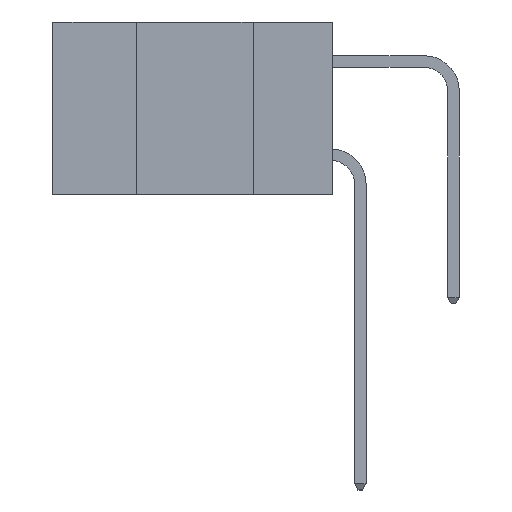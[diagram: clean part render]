
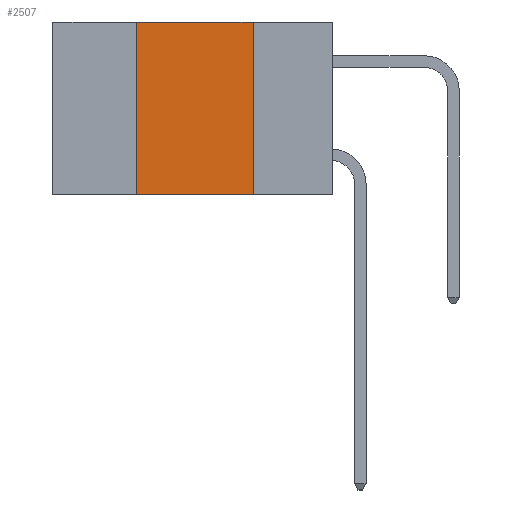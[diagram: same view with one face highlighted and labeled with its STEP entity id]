
A CAD part, left-side view. The second image highlights one B-rep face of the part: STEP entity #2507.
In plain terms, the highlighted planar face has unit normal (-1, 0, 0).
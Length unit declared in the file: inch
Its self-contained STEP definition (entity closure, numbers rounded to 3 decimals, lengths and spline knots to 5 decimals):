
#101 = DIRECTION ( 'NONE',  ( 0., 0., -1. ) ) ;
#121 = DIRECTION ( 'NONE',  ( 1., 0., 0. ) ) ;
#188 = PLANE ( 'NONE',  #5270 ) ;
#397 = CARTESIAN_POINT ( 'NONE',  ( 0., 0.42, -0.37 ) ) ;
#451 = CARTESIAN_POINT ( 'NONE',  ( 0., 0.6, 0. ) ) ;
#1336 = VERTEX_POINT ( 'NONE', #10662 ) ;
#1755 = VECTOR ( 'NONE', #9668, 39.37008 ) ;
#2388 = LINE ( 'NONE', #8891, #1755 ) ;
#2507 = ADVANCED_FACE ( 'NONE', ( #6720 ), #188, .F. ) ;
#2971 = CARTESIAN_POINT ( 'NONE',  ( 0., 0.42, -0.37 ) ) ;
#2998 = VECTOR ( 'NONE', #10975, 39.37008 ) ;
#3882 = VERTEX_POINT ( 'NONE', #397 ) ;
#4764 = ORIENTED_EDGE ( 'NONE', *, *, #8231, .F. ) ;
#5189 = VERTEX_POINT ( 'NONE', #8303 ) ;
#5270 = AXIS2_PLACEMENT_3D ( 'NONE', #451, #121, #101 ) ;
#5668 = LINE ( 'NONE', #7207, #2998 ) ;
#6447 = DIRECTION ( 'NONE',  ( 0., 0., -1. ) ) ;
#6545 = DIRECTION ( 'NONE',  ( 0., 0., 1. ) ) ;
#6720 = FACE_OUTER_BOUND ( 'NONE', #9054, .T. ) ;
#7035 = ORIENTED_EDGE ( 'NONE', *, *, #8243, .F. ) ;
#7207 = CARTESIAN_POINT ( 'NONE',  ( 0., 0.6, 0. ) ) ;
#7280 = VERTEX_POINT ( 'NONE', #8257 ) ;
#7554 = VECTOR ( 'NONE', #6447, 39.37008 ) ;
#8231 = EDGE_CURVE ( 'NONE', #1336, #7280, #9837, .T. ) ;
#8243 = EDGE_CURVE ( 'NONE', #5189, #1336, #5668, .T. ) ;
#8257 = CARTESIAN_POINT ( 'NONE',  ( 0., 0.17, -0.37 ) ) ;
#8303 = CARTESIAN_POINT ( 'NONE',  ( 0., 0.42, 0. ) ) ;
#8430 = EDGE_CURVE ( 'NONE', #3882, #5189, #10858, .T. ) ;
#8520 = EDGE_CURVE ( 'NONE', #3882, #7280, #2388, .T. ) ;
#8877 = VECTOR ( 'NONE', #6545, 39.37008 ) ;
#8891 = CARTESIAN_POINT ( 'NONE',  ( 0., 0.6, -0.37 ) ) ;
#9054 = EDGE_LOOP ( 'NONE', ( #4764, #7035, #9086, #9323 ) ) ;
#9086 = ORIENTED_EDGE ( 'NONE', *, *, #8430, .F. ) ;
#9323 = ORIENTED_EDGE ( 'NONE', *, *, #8520, .T. ) ;
#9668 = DIRECTION ( 'NONE',  ( 0., -1., 0. ) ) ;
#9837 = LINE ( 'NONE', #10234, #7554 ) ;
#10234 = CARTESIAN_POINT ( 'NONE',  ( 0., 0.17, -0.37 ) ) ;
#10662 = CARTESIAN_POINT ( 'NONE',  ( 0., 0.17, 0. ) ) ;
#10858 = LINE ( 'NONE', #2971, #8877 ) ;
#10975 = DIRECTION ( 'NONE',  ( 0., -1., 0. ) ) ;
